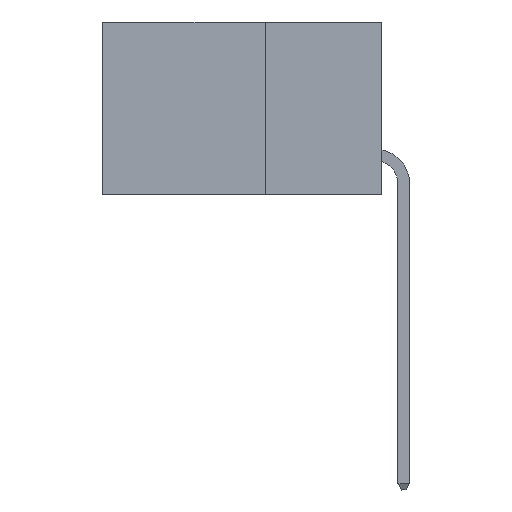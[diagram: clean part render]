
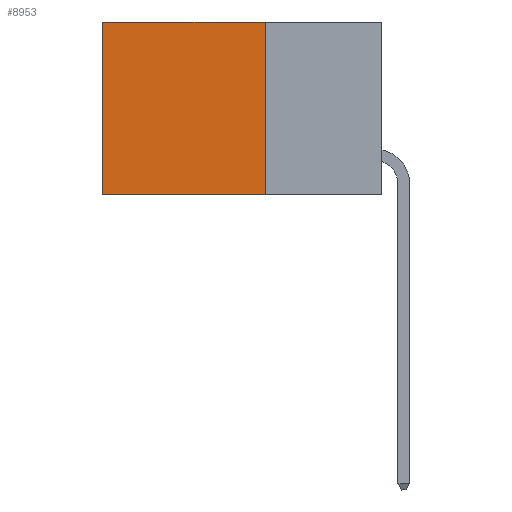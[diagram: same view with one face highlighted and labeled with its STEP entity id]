
A CAD part, left-side view. The second image highlights one B-rep face of the part: STEP entity #8953.
In plain terms, the highlighted planar face has unit normal (-1, 0, 0).
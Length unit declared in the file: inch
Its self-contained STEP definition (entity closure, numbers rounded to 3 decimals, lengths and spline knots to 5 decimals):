
#168 = CARTESIAN_POINT ( 'NONE',  ( 0.2875, 0.25, 0. ) ) ;
#245 = DIRECTION ( 'NONE',  ( 1., 0., 0. ) ) ;
#1073 = ORIENTED_EDGE ( 'NONE', *, *, #6512, .F. ) ;
#1456 = DIRECTION ( 'NONE',  ( 0., 0., -1. ) ) ;
#1503 = EDGE_LOOP ( 'NONE', ( #3365, #11115, #1073, #11056 ) ) ;
#2209 = CARTESIAN_POINT ( 'NONE',  ( 0.2875, 0.25, 0. ) ) ;
#2644 = DIRECTION ( 'NONE',  ( 0., 0., -1. ) ) ;
#2660 = VERTEX_POINT ( 'NONE', #4926 ) ;
#2923 = LINE ( 'NONE', #15514, #5939 ) ;
#3297 = CARTESIAN_POINT ( 'NONE',  ( 0.2875, 0.25, -0.37 ) ) ;
#3365 = ORIENTED_EDGE ( 'NONE', *, *, #14244, .T. ) ;
#4222 = LINE ( 'NONE', #2209, #13049 ) ;
#4484 = EDGE_CURVE ( 'NONE', #8561, #2660, #11137, .T. ) ;
#4926 = CARTESIAN_POINT ( 'NONE',  ( 0.2875, 0.6, -0.37 ) ) ;
#5033 = CARTESIAN_POINT ( 'NONE',  ( 0.2875, 0.25, 0. ) ) ;
#5390 = CARTESIAN_POINT ( 'NONE',  ( 0.2875, 0.25, 0. ) ) ;
#5939 = VECTOR ( 'NONE', #7020, 39.37008 ) ;
#6512 = EDGE_CURVE ( 'NONE', #8000, #8561, #14290, .T. ) ;
#7020 = DIRECTION ( 'NONE',  ( 0., 0., -1. ) ) ;
#7854 = CARTESIAN_POINT ( 'NONE',  ( 0.2875, 0.6, 0. ) ) ;
#8000 = VERTEX_POINT ( 'NONE', #5390 ) ;
#8044 = DIRECTION ( 'NONE',  ( 0., 1., 0. ) ) ;
#8341 = FACE_OUTER_BOUND ( 'NONE', #1503, .T. ) ;
#8561 = VERTEX_POINT ( 'NONE', #8873 ) ;
#8873 = CARTESIAN_POINT ( 'NONE',  ( 0.2875, 0.25, -0.37 ) ) ;
#8953 = ADVANCED_FACE ( 'NONE', ( #8341 ), #9706, .F. ) ;
#9706 = PLANE ( 'NONE',  #12532 ) ;
#10149 = VECTOR ( 'NONE', #2644, 39.37008 ) ;
#10609 = DIRECTION ( 'NONE',  ( 0., 1., 0. ) ) ;
#11056 = ORIENTED_EDGE ( 'NONE', *, *, #14224, .T. ) ;
#11115 = ORIENTED_EDGE ( 'NONE', *, *, #4484, .F. ) ;
#11137 = LINE ( 'NONE', #3297, #13979 ) ;
#11784 = VERTEX_POINT ( 'NONE', #7854 ) ;
#12532 = AXIS2_PLACEMENT_3D ( 'NONE', #5033, #245, #1456 ) ;
#13049 = VECTOR ( 'NONE', #10609, 39.37008 ) ;
#13979 = VECTOR ( 'NONE', #8044, 39.37008 ) ;
#14224 = EDGE_CURVE ( 'NONE', #8000, #11784, #4222, .T. ) ;
#14244 = EDGE_CURVE ( 'NONE', #11784, #2660, #2923, .T. ) ;
#14290 = LINE ( 'NONE', #168, #10149 ) ;
#15514 = CARTESIAN_POINT ( 'NONE',  ( 0.2875, 0.6, 0. ) ) ;
